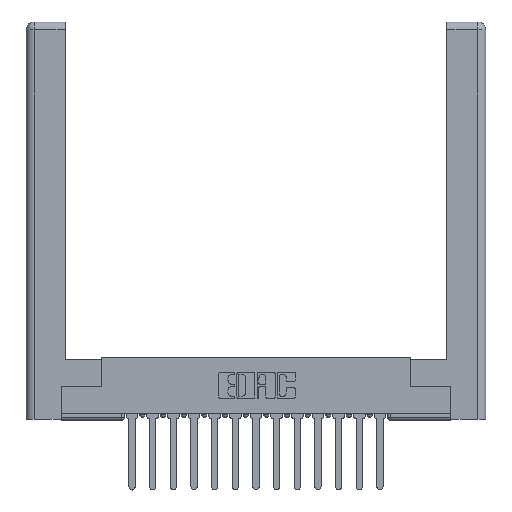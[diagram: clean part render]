
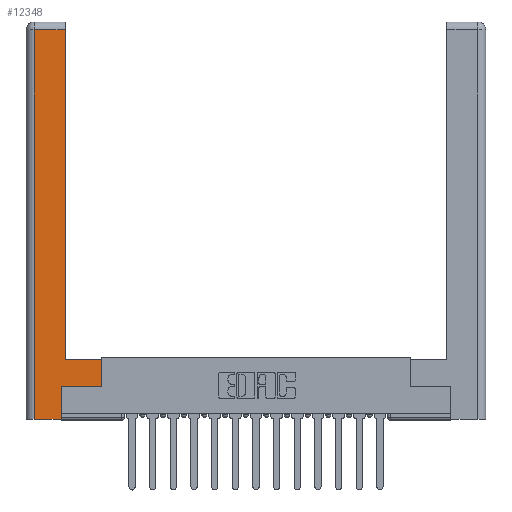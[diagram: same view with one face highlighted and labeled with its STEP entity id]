
A CAD part, top view. The second image highlights one B-rep face of the part: STEP entity #12348.
In plain terms, the highlighted planar face has unit normal (0, 0, 1).
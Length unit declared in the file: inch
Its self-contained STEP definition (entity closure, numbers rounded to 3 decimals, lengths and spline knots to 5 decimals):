
#400 = CARTESIAN_POINT ( 'NONE',  ( 0.295, 0.45, 0. ) ) ;
#1012 = DIRECTION ( 'NONE',  ( 0., -1., 0. ) ) ;
#1144 = ORIENTED_EDGE ( 'NONE', *, *, #10148, .T. ) ;
#1151 = ORIENTED_EDGE ( 'NONE', *, *, #2234, .T. ) ;
#1364 = PLANE ( 'NONE',  #16765 ) ;
#1603 = VECTOR ( 'NONE', #9873, 39.37008 ) ;
#1774 = VECTOR ( 'NONE', #14137, 39.37008 ) ;
#2153 = ORIENTED_EDGE ( 'NONE', *, *, #8778, .T. ) ;
#2179 = CARTESIAN_POINT ( 'NONE',  ( 0.295, 0.45, 0. ) ) ;
#2234 = EDGE_CURVE ( 'NONE', #3636, #16522, #8861, .T. ) ;
#2240 = EDGE_CURVE ( 'NONE', #9323, #16833, #14662, .T. ) ;
#2825 = DIRECTION ( 'NONE',  ( 0., 1., 0. ) ) ;
#3270 = CARTESIAN_POINT ( 'NONE',  ( 0.265, 0., 0. ) ) ;
#3636 = VERTEX_POINT ( 'NONE', #9567 ) ;
#4017 = ORIENTED_EDGE ( 'NONE', *, *, #16313, .T. ) ;
#4654 = ORIENTED_EDGE ( 'NONE', *, *, #2240, .T. ) ;
#4834 = LINE ( 'NONE', #10584, #9417 ) ;
#5284 = CARTESIAN_POINT ( 'NONE',  ( 0.0615, 0., 0. ) ) ;
#5335 = LINE ( 'NONE', #9978, #1774 ) ;
#5521 = CARTESIAN_POINT ( 'NONE',  ( 0.565, 0.245, 0. ) ) ;
#7109 = CARTESIAN_POINT ( 'NONE',  ( 0.0615, 2.94, 0. ) ) ;
#7371 = LINE ( 'NONE', #14251, #9218 ) ;
#7440 = DIRECTION ( 'NONE',  ( 0., 1., 0. ) ) ;
#8778 = EDGE_CURVE ( 'NONE', #11999, #14953, #13655, .T. ) ;
#8861 = LINE ( 'NONE', #9694, #11337 ) ;
#8973 = VERTEX_POINT ( 'NONE', #9761 ) ;
#9218 = VECTOR ( 'NONE', #7440, 39.37008 ) ;
#9323 = VERTEX_POINT ( 'NONE', #17167 ) ;
#9326 = EDGE_LOOP ( 'NONE', ( #4017, #10479, #2153, #1144, #14967, #1151, #14153, #4654 ) ) ;
#9417 = VECTOR ( 'NONE', #2825, 39.37008 ) ;
#9567 = CARTESIAN_POINT ( 'NONE',  ( 0.265, 0.245, 0. ) ) ;
#9586 = EDGE_CURVE ( 'NONE', #16522, #9323, #5335, .T. ) ;
#9592 = DIRECTION ( 'NONE',  ( 1., 0., 0. ) ) ;
#9694 = CARTESIAN_POINT ( 'NONE',  ( 0.565, 0.245, 0. ) ) ;
#9761 = CARTESIAN_POINT ( 'NONE',  ( 0.295, 2.94, 0. ) ) ;
#9873 = DIRECTION ( 'NONE',  ( -1., 0., 0. ) ) ;
#9978 = CARTESIAN_POINT ( 'NONE',  ( 0.565, 0.45, 0. ) ) ;
#10148 = EDGE_CURVE ( 'NONE', #14953, #12023, #13837, .T. ) ;
#10177 = LINE ( 'NONE', #7109, #1603 ) ;
#10479 = ORIENTED_EDGE ( 'NONE', *, *, #13078, .T. ) ;
#10536 = VECTOR ( 'NONE', #13815, 39.37008 ) ;
#10584 = CARTESIAN_POINT ( 'NONE',  ( 0.295, 3., 0. ) ) ;
#10657 = CARTESIAN_POINT ( 'NONE',  ( 0., 0., 0. ) ) ;
#11337 = VECTOR ( 'NONE', #9592, 39.37008 ) ;
#11941 = FACE_OUTER_BOUND ( 'NONE', #9326, .T. ) ;
#11993 = DIRECTION ( 'NONE',  ( 0., 0., -1. ) ) ;
#11999 = VERTEX_POINT ( 'NONE', #15571 ) ;
#12023 = VERTEX_POINT ( 'NONE', #12973 ) ;
#12073 = EDGE_CURVE ( 'NONE', #12023, #3636, #7371, .T. ) ;
#12348 = ADVANCED_FACE ( 'NONE', ( #11941 ), #1364, .F. ) ;
#12881 = CARTESIAN_POINT ( 'NONE',  ( 0.0615, 0., 0. ) ) ;
#12973 = CARTESIAN_POINT ( 'NONE',  ( 0.265, 0., 0. ) ) ;
#13078 = EDGE_CURVE ( 'NONE', #8973, #11999, #10177, .T. ) ;
#13655 = LINE ( 'NONE', #5284, #14710 ) ;
#13787 = DIRECTION ( 'NONE',  ( -1., 0., 0. ) ) ;
#13815 = DIRECTION ( 'NONE',  ( 1., 0., 0. ) ) ;
#13837 = LINE ( 'NONE', #3270, #10536 ) ;
#14137 = DIRECTION ( 'NONE',  ( 0., 1., 0. ) ) ;
#14153 = ORIENTED_EDGE ( 'NONE', *, *, #9586, .T. ) ;
#14251 = CARTESIAN_POINT ( 'NONE',  ( 0.265, 0.245, 0. ) ) ;
#14662 = LINE ( 'NONE', #400, #15747 ) ;
#14710 = VECTOR ( 'NONE', #1012, 39.37008 ) ;
#14953 = VERTEX_POINT ( 'NONE', #12881 ) ;
#14967 = ORIENTED_EDGE ( 'NONE', *, *, #12073, .T. ) ;
#15020 = DIRECTION ( 'NONE',  ( -1., 0., 0. ) ) ;
#15571 = CARTESIAN_POINT ( 'NONE',  ( 0.0615, 2.94, 0. ) ) ;
#15747 = VECTOR ( 'NONE', #13787, 39.37008 ) ;
#16313 = EDGE_CURVE ( 'NONE', #16833, #8973, #4834, .T. ) ;
#16522 = VERTEX_POINT ( 'NONE', #5521 ) ;
#16765 = AXIS2_PLACEMENT_3D ( 'NONE', #10657, #11993, #15020 ) ;
#16833 = VERTEX_POINT ( 'NONE', #2179 ) ;
#17167 = CARTESIAN_POINT ( 'NONE',  ( 0.565, 0.45, 0. ) ) ;
